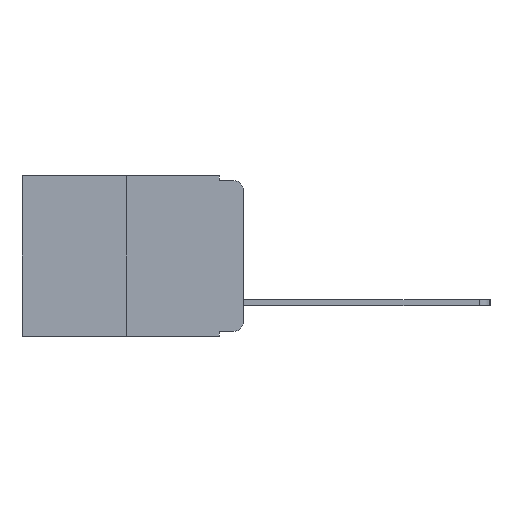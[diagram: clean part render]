
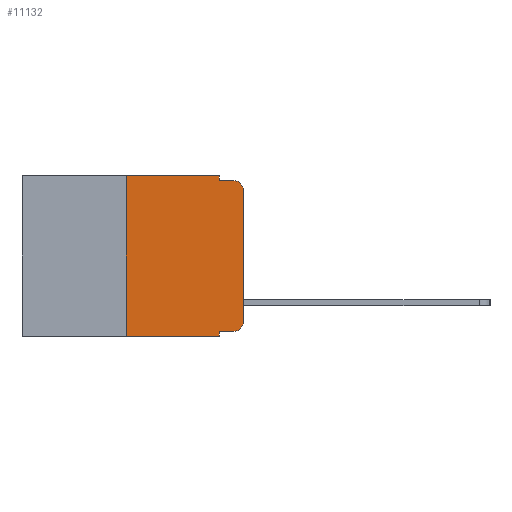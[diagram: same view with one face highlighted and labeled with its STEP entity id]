
A CAD part, left-side view. The second image highlights one B-rep face of the part: STEP entity #11132.
In plain terms, the highlighted planar face has unit normal (-1, 0, 0).
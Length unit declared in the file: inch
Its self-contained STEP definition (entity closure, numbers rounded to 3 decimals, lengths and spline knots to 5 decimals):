
#57 = LINE ( 'NONE', #10537, #2761 ) ;
#117 = ORIENTED_EDGE ( 'NONE', *, *, #3577, .F. ) ;
#163 = ORIENTED_EDGE ( 'NONE', *, *, #9221, .T. ) ;
#225 = EDGE_CURVE ( 'NONE', #10153, #8595, #4388, .T. ) ;
#430 = CARTESIAN_POINT ( 'NONE',  ( 0., 0.02, -0.333 ) ) ;
#625 = ORIENTED_EDGE ( 'NONE', *, *, #225, .F. ) ;
#695 = VECTOR ( 'NONE', #9969, 39.37008 ) ;
#997 = DIRECTION ( 'NONE',  ( 0., -1., 0. ) ) ;
#1085 = VERTEX_POINT ( 'NONE', #8138 ) ;
#1145 = DIRECTION ( 'NONE',  ( 0., 0., -1. ) ) ;
#1234 = CARTESIAN_POINT ( 'NONE',  ( 0., 0., -0.313 ) ) ;
#1268 = CARTESIAN_POINT ( 'NONE',  ( 0., 0.051, -0.333 ) ) ;
#1337 = VERTEX_POINT ( 'NONE', #1234 ) ;
#1340 = VECTOR ( 'NONE', #997, 39.37008 ) ;
#1581 = CIRCLE ( 'NONE', #6334, 0.02 ) ;
#1887 = DIRECTION ( 'NONE',  ( -1., 0., 0. ) ) ;
#1969 = DIRECTION ( 'NONE',  ( 0., -1., 0. ) ) ;
#2074 = LINE ( 'NONE', #5359, #12700 ) ;
#2251 = CARTESIAN_POINT ( 'NONE',  ( 0., 0., 0. ) ) ;
#2340 = CARTESIAN_POINT ( 'NONE',  ( 0., 0.051, 0. ) ) ;
#2377 = EDGE_CURVE ( 'NONE', #12311, #8609, #2648, .T. ) ;
#2444 = EDGE_CURVE ( 'NONE', #5831, #6630, #1581, .T. ) ;
#2648 = LINE ( 'NONE', #8607, #11058 ) ;
#2761 = VECTOR ( 'NONE', #7286, 39.37008 ) ;
#2767 = CARTESIAN_POINT ( 'NONE',  ( 0., 0.02, -0.01 ) ) ;
#2775 = CARTESIAN_POINT ( 'NONE',  ( 0., 0.051, 0. ) ) ;
#2887 = VECTOR ( 'NONE', #8969, 39.37008 ) ;
#3356 = ORIENTED_EDGE ( 'NONE', *, *, #7032, .T. ) ;
#3475 = ORIENTED_EDGE ( 'NONE', *, *, #9836, .F. ) ;
#3577 = EDGE_CURVE ( 'NONE', #1085, #12311, #2074, .T. ) ;
#3983 = ORIENTED_EDGE ( 'NONE', *, *, #2444, .T. ) ;
#4333 = LINE ( 'NONE', #10919, #1340 ) ;
#4388 = LINE ( 'NONE', #11564, #4744 ) ;
#4449 = LINE ( 'NONE', #1268, #12784 ) ;
#4491 = DIRECTION ( 'NONE',  ( 0., 0., -1. ) ) ;
#4685 = DIRECTION ( 'NONE',  ( 0., -1., 0. ) ) ;
#4744 = VECTOR ( 'NONE', #11619, 39.37008 ) ;
#5359 = CARTESIAN_POINT ( 'NONE',  ( 0., 0.25, 0. ) ) ;
#5624 = ORIENTED_EDGE ( 'NONE', *, *, #9737, .T. ) ;
#5831 = VERTEX_POINT ( 'NONE', #5886 ) ;
#5875 = LINE ( 'NONE', #2340, #2887 ) ;
#5886 = CARTESIAN_POINT ( 'NONE',  ( 0., 0., -0.03 ) ) ;
#6334 = AXIS2_PLACEMENT_3D ( 'NONE', #14254, #7838, #1145 ) ;
#6367 = LINE ( 'NONE', #2251, #695 ) ;
#6552 = ORIENTED_EDGE ( 'NONE', *, *, #11186, .F. ) ;
#6572 = FACE_OUTER_BOUND ( 'NONE', #13342, .T. ) ;
#6630 = VERTEX_POINT ( 'NONE', #2767 ) ;
#7032 = EDGE_CURVE ( 'NONE', #10153, #11903, #4449, .T. ) ;
#7091 = ORIENTED_EDGE ( 'NONE', *, *, #12257, .T. ) ;
#7149 = CIRCLE ( 'NONE', #8309, 0.02 ) ;
#7150 = CARTESIAN_POINT ( 'NONE',  ( 0., 0.051, -0.333 ) ) ;
#7286 = DIRECTION ( 'NONE',  ( 0., -1., 0. ) ) ;
#7588 = DIRECTION ( 'NONE',  ( 0., 0., 1. ) ) ;
#7838 = DIRECTION ( 'NONE',  ( -1., 0., 0. ) ) ;
#8138 = CARTESIAN_POINT ( 'NONE',  ( 0., 0.25, -0.343 ) ) ;
#8193 = VERTEX_POINT ( 'NONE', #11940 ) ;
#8309 = AXIS2_PLACEMENT_3D ( 'NONE', #8517, #1887, #9622 ) ;
#8517 = CARTESIAN_POINT ( 'NONE',  ( 0., 0.02, -0.313 ) ) ;
#8595 = VERTEX_POINT ( 'NONE', #10475 ) ;
#8607 = CARTESIAN_POINT ( 'NONE',  ( 0., 0.473, 0. ) ) ;
#8609 = VERTEX_POINT ( 'NONE', #2775 ) ;
#8806 = ORIENTED_EDGE ( 'NONE', *, *, #2377, .F. ) ;
#8869 = CARTESIAN_POINT ( 'NONE',  ( 0., 0.473, 0. ) ) ;
#8969 = DIRECTION ( 'NONE',  ( 0., 0., -1. ) ) ;
#9221 = EDGE_CURVE ( 'NONE', #11903, #1337, #7149, .T. ) ;
#9338 = AXIS2_PLACEMENT_3D ( 'NONE', #8869, #11025, #4491 ) ;
#9622 = DIRECTION ( 'NONE',  ( 0., 0., -1. ) ) ;
#9737 = EDGE_CURVE ( 'NONE', #1085, #8595, #57, .T. ) ;
#9836 = EDGE_CURVE ( 'NONE', #8193, #6630, #4333, .T. ) ;
#9954 = PLANE ( 'NONE',  #9338 ) ;
#9969 = DIRECTION ( 'NONE',  ( 0., 0., 1. ) ) ;
#10016 = CARTESIAN_POINT ( 'NONE',  ( 0., 0.25, 0. ) ) ;
#10153 = VERTEX_POINT ( 'NONE', #7150 ) ;
#10475 = CARTESIAN_POINT ( 'NONE',  ( 0., 0.051, -0.343 ) ) ;
#10537 = CARTESIAN_POINT ( 'NONE',  ( 0., 0.473, -0.343 ) ) ;
#10919 = CARTESIAN_POINT ( 'NONE',  ( 0., 0.051, -0.01 ) ) ;
#11025 = DIRECTION ( 'NONE',  ( 1., 0., 0. ) ) ;
#11058 = VECTOR ( 'NONE', #1969, 39.37008 ) ;
#11132 = ADVANCED_FACE ( 'NONE', ( #6572 ), #9954, .F. ) ;
#11186 = EDGE_CURVE ( 'NONE', #8609, #8193, #5875, .T. ) ;
#11564 = CARTESIAN_POINT ( 'NONE',  ( 0., 0.051, 0. ) ) ;
#11619 = DIRECTION ( 'NONE',  ( 0., 0., -1. ) ) ;
#11903 = VERTEX_POINT ( 'NONE', #430 ) ;
#11940 = CARTESIAN_POINT ( 'NONE',  ( 0., 0.051, -0.01 ) ) ;
#12257 = EDGE_CURVE ( 'NONE', #1337, #5831, #6367, .T. ) ;
#12311 = VERTEX_POINT ( 'NONE', #10016 ) ;
#12700 = VECTOR ( 'NONE', #7588, 39.37008 ) ;
#12784 = VECTOR ( 'NONE', #4685, 39.37008 ) ;
#13342 = EDGE_LOOP ( 'NONE', ( #7091, #3983, #3475, #6552, #8806, #117, #5624, #625, #3356, #163 ) ) ;
#14254 = CARTESIAN_POINT ( 'NONE',  ( 0., 0.02, -0.03 ) ) ;
